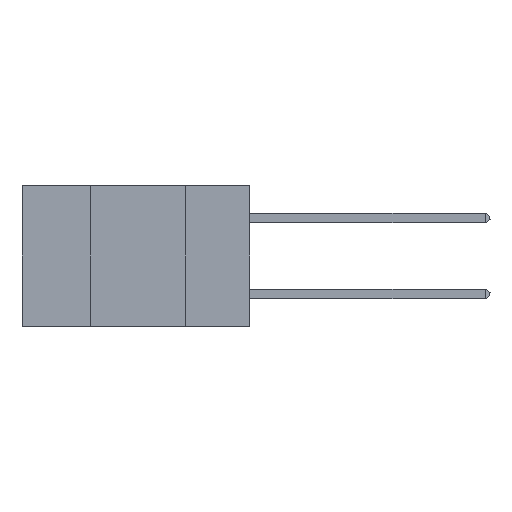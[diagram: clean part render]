
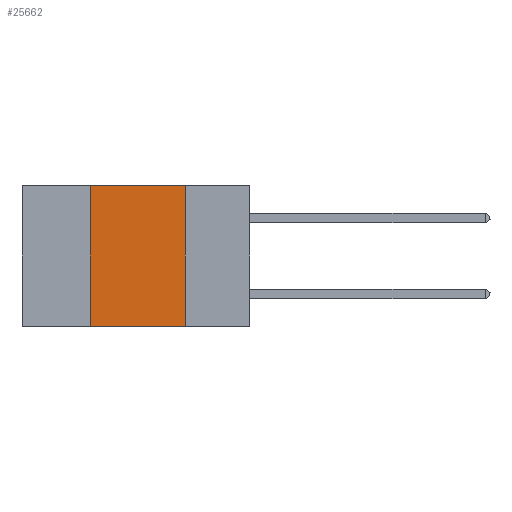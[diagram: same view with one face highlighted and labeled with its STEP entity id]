
A CAD part, left-side view. The second image highlights one B-rep face of the part: STEP entity #25662.
In plain terms, the highlighted planar face has unit normal (-1, 0, 0).
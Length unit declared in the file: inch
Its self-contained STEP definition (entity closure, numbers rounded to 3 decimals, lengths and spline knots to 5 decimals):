
#2162 = EDGE_CURVE ( 'NONE', #31754, #16890, #7540, .T. ) ;
#3444 = VECTOR ( 'NONE', #24447, 39.37008 ) ;
#5743 = CARTESIAN_POINT ( 'NONE',  ( 0., 0.42, 0. ) ) ;
#5822 = EDGE_CURVE ( 'NONE', #21428, #15576, #14163, .T. ) ;
#5823 = ORIENTED_EDGE ( 'NONE', *, *, #34126, .F. ) ;
#6831 = CARTESIAN_POINT ( 'NONE',  ( 0., 0.6, 0. ) ) ;
#6978 = DIRECTION ( 'NONE',  ( 0., 0., -1. ) ) ;
#7227 = DIRECTION ( 'NONE',  ( 0., -1., 0. ) ) ;
#7398 = FACE_OUTER_BOUND ( 'NONE', #37566, .T. ) ;
#7540 = LINE ( 'NONE', #16131, #38882 ) ;
#9111 = VECTOR ( 'NONE', #7227, 39.37008 ) ;
#9954 = DIRECTION ( 'NONE',  ( 0., 0., -1. ) ) ;
#11292 = CARTESIAN_POINT ( 'NONE',  ( 0., 0.42, -0.37 ) ) ;
#11735 = LINE ( 'NONE', #39457, #3444 ) ;
#14163 = LINE ( 'NONE', #5743, #22257 ) ;
#15576 = VERTEX_POINT ( 'NONE', #33512 ) ;
#15950 = ORIENTED_EDGE ( 'NONE', *, *, #5822, .F. ) ;
#15992 = PLANE ( 'NONE',  #25307 ) ;
#16131 = CARTESIAN_POINT ( 'NONE',  ( 0., 0.17, 0. ) ) ;
#16890 = VERTEX_POINT ( 'NONE', #36631 ) ;
#21428 = VERTEX_POINT ( 'NONE', #11292 ) ;
#22257 = VECTOR ( 'NONE', #30136, 39.37008 ) ;
#24040 = ORIENTED_EDGE ( 'NONE', *, *, #26229, .T. ) ;
#24447 = DIRECTION ( 'NONE',  ( 0., -1., 0. ) ) ;
#25307 = AXIS2_PLACEMENT_3D ( 'NONE', #6831, #28147, #9954 ) ;
#25662 = ADVANCED_FACE ( 'NONE', ( #7398 ), #15992, .F. ) ;
#26229 = EDGE_CURVE ( 'NONE', #21428, #16890, #11735, .T. ) ;
#28147 = DIRECTION ( 'NONE',  ( 1., 0., 0. ) ) ;
#28534 = CARTESIAN_POINT ( 'NONE',  ( 0., 0.6, 0. ) ) ;
#29181 = ORIENTED_EDGE ( 'NONE', *, *, #2162, .F. ) ;
#30136 = DIRECTION ( 'NONE',  ( 0., 0., 1. ) ) ;
#31754 = VERTEX_POINT ( 'NONE', #38167 ) ;
#33327 = LINE ( 'NONE', #28534, #9111 ) ;
#33512 = CARTESIAN_POINT ( 'NONE',  ( 0., 0.42, 0. ) ) ;
#34126 = EDGE_CURVE ( 'NONE', #15576, #31754, #33327, .T. ) ;
#36631 = CARTESIAN_POINT ( 'NONE',  ( 0., 0.17, -0.37 ) ) ;
#37566 = EDGE_LOOP ( 'NONE', ( #29181, #5823, #15950, #24040 ) ) ;
#38167 = CARTESIAN_POINT ( 'NONE',  ( 0., 0.17, 0. ) ) ;
#38882 = VECTOR ( 'NONE', #6978, 39.37008 ) ;
#39457 = CARTESIAN_POINT ( 'NONE',  ( 0., 0.6, -0.37 ) ) ;
